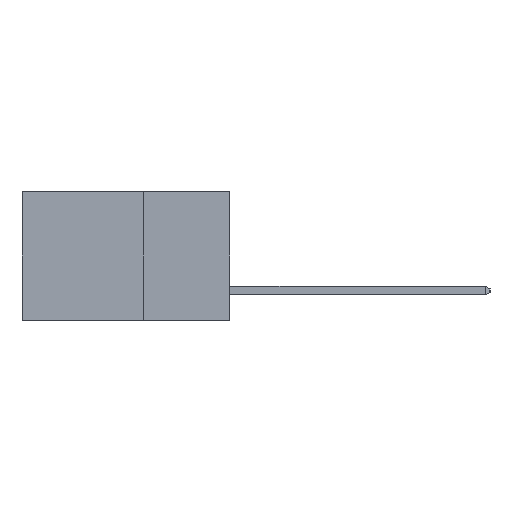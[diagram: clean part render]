
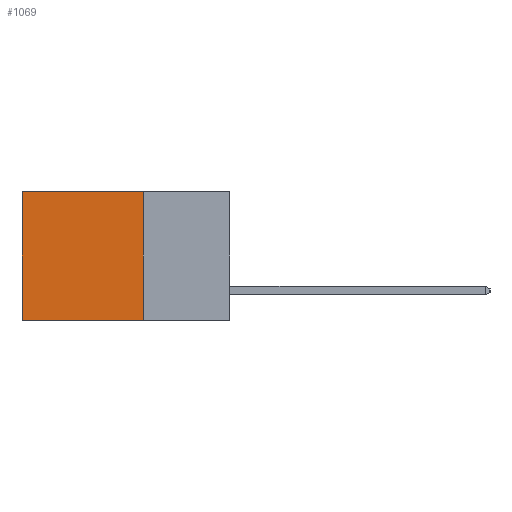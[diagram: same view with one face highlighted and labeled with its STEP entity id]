
A CAD part, left-side view. The second image highlights one B-rep face of the part: STEP entity #1069.
In plain terms, the highlighted planar face has unit normal (-1, 0, 0).
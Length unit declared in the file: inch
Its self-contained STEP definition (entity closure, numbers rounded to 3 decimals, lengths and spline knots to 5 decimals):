
#82 = DIRECTION ( 'NONE',  ( 0., 0., -1. ) ) ;
#871 = PLANE ( 'NONE',  #4459 ) ;
#939 = CARTESIAN_POINT ( 'NONE',  ( 0.298, 0.25, 0. ) ) ;
#1069 = ADVANCED_FACE ( 'NONE', ( #10284 ), #871, .F. ) ;
#1279 = VERTEX_POINT ( 'NONE', #10153 ) ;
#1482 = EDGE_CURVE ( 'NONE', #13282, #7777, #10850, .T. ) ;
#1667 = LINE ( 'NONE', #11994, #7894 ) ;
#1805 = LINE ( 'NONE', #6350, #13778 ) ;
#2001 = DIRECTION ( 'NONE',  ( 0., 1., 0. ) ) ;
#2395 = CARTESIAN_POINT ( 'NONE',  ( 0.298, 0.25, -0.37 ) ) ;
#2617 = ORIENTED_EDGE ( 'NONE', *, *, #7373, .F. ) ;
#2713 = DIRECTION ( 'NONE',  ( 0., 0., -1. ) ) ;
#2940 = CARTESIAN_POINT ( 'NONE',  ( 0.298, 0.25, 0. ) ) ;
#2995 = EDGE_CURVE ( 'NONE', #13282, #1279, #6660, .T. ) ;
#3337 = CARTESIAN_POINT ( 'NONE',  ( 0.298, 0.25, 0. ) ) ;
#4230 = ORIENTED_EDGE ( 'NONE', *, *, #2995, .T. ) ;
#4459 = AXIS2_PLACEMENT_3D ( 'NONE', #939, #14462, #9810 ) ;
#6350 = CARTESIAN_POINT ( 'NONE',  ( 0.298, 0.25, -0.37 ) ) ;
#6384 = ORIENTED_EDGE ( 'NONE', *, *, #1482, .F. ) ;
#6660 = LINE ( 'NONE', #3337, #12443 ) ;
#7373 = EDGE_CURVE ( 'NONE', #7777, #11340, #1805, .T. ) ;
#7777 = VERTEX_POINT ( 'NONE', #2395 ) ;
#7894 = VECTOR ( 'NONE', #2713, 39.37008 ) ;
#8123 = VECTOR ( 'NONE', #82, 39.37008 ) ;
#8506 = CARTESIAN_POINT ( 'NONE',  ( 0.298, 0.25, 0. ) ) ;
#9152 = ORIENTED_EDGE ( 'NONE', *, *, #14813, .T. ) ;
#9642 = EDGE_LOOP ( 'NONE', ( #9152, #2617, #6384, #4230 ) ) ;
#9810 = DIRECTION ( 'NONE',  ( 0., 0., -1. ) ) ;
#10153 = CARTESIAN_POINT ( 'NONE',  ( 0.298, 0.6, 0. ) ) ;
#10284 = FACE_OUTER_BOUND ( 'NONE', #9642, .T. ) ;
#10850 = LINE ( 'NONE', #8506, #8123 ) ;
#11340 = VERTEX_POINT ( 'NONE', #14654 ) ;
#11994 = CARTESIAN_POINT ( 'NONE',  ( 0.298, 0.6, 0. ) ) ;
#12109 = DIRECTION ( 'NONE',  ( 0., 1., 0. ) ) ;
#12443 = VECTOR ( 'NONE', #2001, 39.37008 ) ;
#13282 = VERTEX_POINT ( 'NONE', #2940 ) ;
#13778 = VECTOR ( 'NONE', #12109, 39.37008 ) ;
#14462 = DIRECTION ( 'NONE',  ( 1., 0., 0. ) ) ;
#14654 = CARTESIAN_POINT ( 'NONE',  ( 0.298, 0.6, -0.37 ) ) ;
#14813 = EDGE_CURVE ( 'NONE', #1279, #11340, #1667, .T. ) ;
